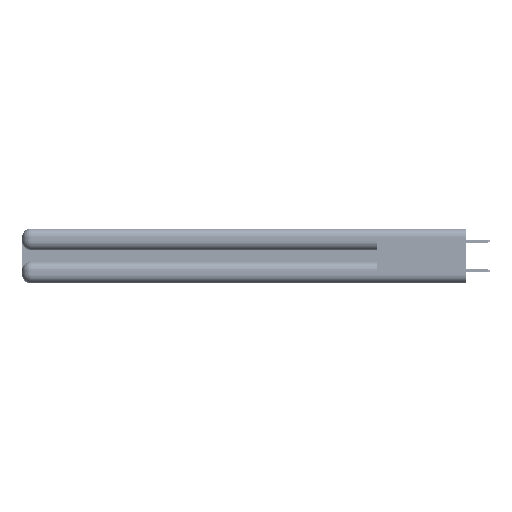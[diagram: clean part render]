
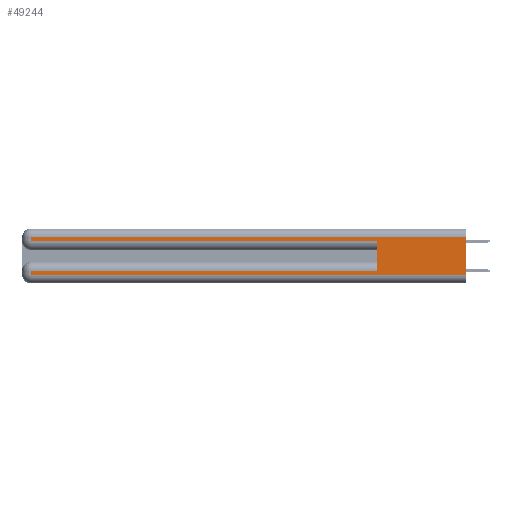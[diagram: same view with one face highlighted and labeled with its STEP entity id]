
A CAD part, left-side view. The second image highlights one B-rep face of the part: STEP entity #49244.
In plain terms, the highlighted planar face has unit normal (-1, 0, 0).
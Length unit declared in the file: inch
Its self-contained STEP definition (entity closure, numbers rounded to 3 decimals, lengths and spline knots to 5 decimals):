
#1055 = DIRECTION ( 'NONE',  ( 0., 0., -1. ) ) ;
#2280 = ORIENTED_EDGE ( 'NONE', *, *, #19577, .T. ) ;
#2872 = VECTOR ( 'NONE', #6558, 39.37008 ) ;
#3274 = CARTESIAN_POINT ( 'NONE',  ( 0., 0., 0.06 ) ) ;
#3702 = VERTEX_POINT ( 'NONE', #24577 ) ;
#4539 = DIRECTION ( 'NONE',  ( 0., 1., 0. ) ) ;
#4566 = EDGE_CURVE ( 'NONE', #26376, #16308, #44337, .T. ) ;
#5052 = EDGE_LOOP ( 'NONE', ( #52799, #6855, #11404, #49357, #37467, #36141, #2280, #17635 ) ) ;
#5214 = CARTESIAN_POINT ( 'NONE',  ( 0., 2.94, 0.085 ) ) ;
#6504 = LINE ( 'NONE', #51711, #27898 ) ;
#6558 = DIRECTION ( 'NONE',  ( 0., -1., 0. ) ) ;
#6855 = ORIENTED_EDGE ( 'NONE', *, *, #33536, .T. ) ;
#6951 = CARTESIAN_POINT ( 'NONE',  ( 0., 2.94, 0.31 ) ) ;
#6986 = AXIS2_PLACEMENT_3D ( 'NONE', #24970, #16555, #46382 ) ;
#7981 = PLANE ( 'NONE',  #6986 ) ;
#9224 = VECTOR ( 'NONE', #1055, 39.37008 ) ;
#11404 = ORIENTED_EDGE ( 'NONE', *, *, #35869, .T. ) ;
#12569 = EDGE_CURVE ( 'NONE', #3702, #17514, #32172, .T. ) ;
#13058 = CARTESIAN_POINT ( 'NONE',  ( 0., 2.94, 0.37 ) ) ;
#13236 = DIRECTION ( 'NONE',  ( 0., 0., -1. ) ) ;
#13422 = CARTESIAN_POINT ( 'NONE',  ( 0., 0., 0.37 ) ) ;
#14204 = LINE ( 'NONE', #27860, #2872 ) ;
#14619 = CARTESIAN_POINT ( 'NONE',  ( 0., 2.94, 0.285 ) ) ;
#15144 = CARTESIAN_POINT ( 'NONE',  ( 0., 0.6, 0.285 ) ) ;
#16308 = VERTEX_POINT ( 'NONE', #15144 ) ;
#16555 = DIRECTION ( 'NONE',  ( 1., 0., 0. ) ) ;
#17514 = VERTEX_POINT ( 'NONE', #20518 ) ;
#17635 = ORIENTED_EDGE ( 'NONE', *, *, #12569, .T. ) ;
#17768 = CARTESIAN_POINT ( 'NONE',  ( 0., 0.6, 0.085 ) ) ;
#18891 = LINE ( 'NONE', #13058, #40301 ) ;
#19577 = EDGE_CURVE ( 'NONE', #40600, #3702, #54510, .T. ) ;
#20518 = CARTESIAN_POINT ( 'NONE',  ( 0., 0., 0.06 ) ) ;
#21624 = DIRECTION ( 'NONE',  ( 0., 0., -1. ) ) ;
#23045 = EDGE_CURVE ( 'NONE', #24322, #16308, #14204, .T. ) ;
#24322 = VERTEX_POINT ( 'NONE', #14619 ) ;
#24577 = CARTESIAN_POINT ( 'NONE',  ( 0., 2.94, 0.06 ) ) ;
#24970 = CARTESIAN_POINT ( 'NONE',  ( 0., 0., 0.37 ) ) ;
#25846 = CARTESIAN_POINT ( 'NONE',  ( 0., 0., 0.085 ) ) ;
#26376 = VERTEX_POINT ( 'NONE', #17768 ) ;
#27028 = LINE ( 'NONE', #25846, #46986 ) ;
#27860 = CARTESIAN_POINT ( 'NONE',  ( 0., 0., 0.285 ) ) ;
#27898 = VECTOR ( 'NONE', #47460, 39.37008 ) ;
#31337 = LINE ( 'NONE', #13422, #42628 ) ;
#31695 = VECTOR ( 'NONE', #52569, 39.37008 ) ;
#32172 = LINE ( 'NONE', #3274, #34841 ) ;
#32530 = VERTEX_POINT ( 'NONE', #6951 ) ;
#33536 = EDGE_CURVE ( 'NONE', #43341, #32530, #6504, .T. ) ;
#34841 = VECTOR ( 'NONE', #50232, 39.37008 ) ;
#35261 = EDGE_CURVE ( 'NONE', #26376, #40600, #27028, .T. ) ;
#35869 = EDGE_CURVE ( 'NONE', #32530, #24322, #18891, .T. ) ;
#36141 = ORIENTED_EDGE ( 'NONE', *, *, #35261, .T. ) ;
#37467 = ORIENTED_EDGE ( 'NONE', *, *, #4566, .F. ) ;
#39806 = CARTESIAN_POINT ( 'NONE',  ( 0., 0.6, 0.145 ) ) ;
#40301 = VECTOR ( 'NONE', #21624, 39.37008 ) ;
#40555 = EDGE_CURVE ( 'NONE', #43341, #17514, #31337, .T. ) ;
#40600 = VERTEX_POINT ( 'NONE', #5214 ) ;
#41859 = FACE_OUTER_BOUND ( 'NONE', #5052, .T. ) ;
#41964 = CARTESIAN_POINT ( 'NONE',  ( 0., 0., 0.31 ) ) ;
#42628 = VECTOR ( 'NONE', #13236, 39.37008 ) ;
#43341 = VERTEX_POINT ( 'NONE', #41964 ) ;
#44337 = LINE ( 'NONE', #39806, #31695 ) ;
#46382 = DIRECTION ( 'NONE',  ( 0., 0., -1. ) ) ;
#46986 = VECTOR ( 'NONE', #4539, 39.37008 ) ;
#47460 = DIRECTION ( 'NONE',  ( 0., 1., 0. ) ) ;
#47867 = CARTESIAN_POINT ( 'NONE',  ( 0., 2.94, 0.37 ) ) ;
#49244 = ADVANCED_FACE ( 'NONE', ( #41859 ), #7981, .F. ) ;
#49357 = ORIENTED_EDGE ( 'NONE', *, *, #23045, .T. ) ;
#50232 = DIRECTION ( 'NONE',  ( 0., -1., 0. ) ) ;
#51711 = CARTESIAN_POINT ( 'NONE',  ( 0., 0., 0.31 ) ) ;
#52569 = DIRECTION ( 'NONE',  ( 0., 0., 1. ) ) ;
#52799 = ORIENTED_EDGE ( 'NONE', *, *, #40555, .F. ) ;
#54510 = LINE ( 'NONE', #47867, #9224 ) ;
